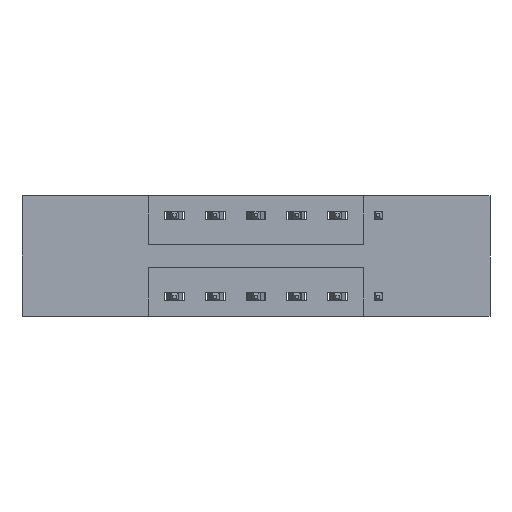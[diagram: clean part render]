
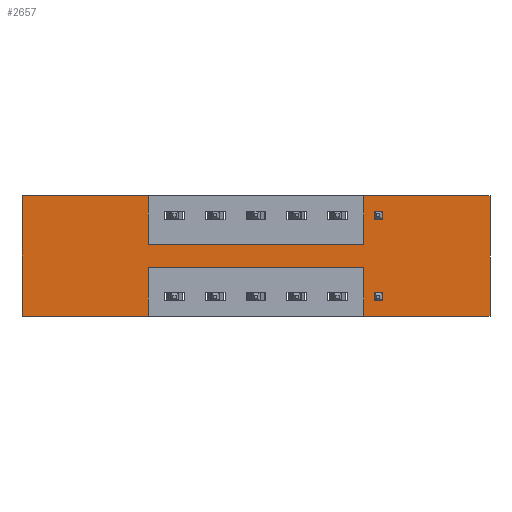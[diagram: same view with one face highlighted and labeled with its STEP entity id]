
A CAD part, front view. The second image highlights one B-rep face of the part: STEP entity #2657.
In plain terms, the highlighted planar face has unit normal (0, -1, 0).
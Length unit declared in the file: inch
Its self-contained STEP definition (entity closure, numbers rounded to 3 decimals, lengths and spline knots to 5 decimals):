
#103 = EDGE_CURVE ( 'NONE', #3690, #7489, #5145, .T. ) ;
#227 = LINE ( 'NONE', #2023, #5489 ) ;
#377 = CARTESIAN_POINT ( 'NONE',  ( 1.0475, 0., -0.37 ) ) ;
#405 = ORIENTED_EDGE ( 'NONE', *, *, #7038, .F. ) ;
#437 = VERTEX_POINT ( 'NONE', #2454 ) ;
#628 = LINE ( 'NONE', #7731, #2457 ) ;
#719 = CARTESIAN_POINT ( 'NONE',  ( 0., 0., -0.37 ) ) ;
#747 = CARTESIAN_POINT ( 'NONE',  ( 0.3875, 0., -0.22 ) ) ;
#749 = EDGE_CURVE ( 'NONE', #3052, #5755, #6843, .T. ) ;
#815 = VECTOR ( 'NONE', #6853, 39.37008 ) ;
#986 = CARTESIAN_POINT ( 'NONE',  ( 0.3875, 0., 0. ) ) ;
#1021 = ORIENTED_EDGE ( 'NONE', *, *, #3793, .F. ) ;
#1059 = LINE ( 'NONE', #377, #2829 ) ;
#1305 = ORIENTED_EDGE ( 'NONE', *, *, #3811, .F. ) ;
#1348 = VECTOR ( 'NONE', #4289, 39.37008 ) ;
#1505 = ORIENTED_EDGE ( 'NONE', *, *, #5177, .F. ) ;
#1814 = CARTESIAN_POINT ( 'NONE',  ( 1.0475, 0., 0. ) ) ;
#1896 = VERTEX_POINT ( 'NONE', #7807 ) ;
#1995 = FACE_OUTER_BOUND ( 'NONE', #5633, .T. ) ;
#2023 = CARTESIAN_POINT ( 'NONE',  ( 0., 0., -0.37 ) ) ;
#2025 = LINE ( 'NONE', #7241, #3007 ) ;
#2126 = EDGE_CURVE ( 'NONE', #5675, #1896, #7620, .T. ) ;
#2211 = EDGE_CURVE ( 'NONE', #4249, #5675, #4907, .T. ) ;
#2221 = DIRECTION ( 'NONE',  ( 1., 0., 0. ) ) ;
#2454 = CARTESIAN_POINT ( 'NONE',  ( 1.435, 0., 0. ) ) ;
#2457 = VECTOR ( 'NONE', #8298, 39.37008 ) ;
#2488 = DIRECTION ( 'NONE',  ( 0., 0., 1. ) ) ;
#2521 = LINE ( 'NONE', #3202, #1348 ) ;
#2657 = ADVANCED_FACE ( 'NONE', ( #1995 ), #7123, .T. ) ;
#2673 = VERTEX_POINT ( 'NONE', #7170 ) ;
#2764 = DIRECTION ( 'NONE',  ( -1., 0., 0. ) ) ;
#2829 = VECTOR ( 'NONE', #3634, 39.37008 ) ;
#2923 = EDGE_CURVE ( 'NONE', #3695, #2673, #227, .T. ) ;
#3007 = VECTOR ( 'NONE', #4045, 39.37008 ) ;
#3041 = VERTEX_POINT ( 'NONE', #747 ) ;
#3052 = VERTEX_POINT ( 'NONE', #8069 ) ;
#3202 = CARTESIAN_POINT ( 'NONE',  ( 0.3875, 0., -0.15 ) ) ;
#3571 = ORIENTED_EDGE ( 'NONE', *, *, #7753, .F. ) ;
#3614 = CARTESIAN_POINT ( 'NONE',  ( 0., 0., 0. ) ) ;
#3634 = DIRECTION ( 'NONE',  ( 0., 0., 1. ) ) ;
#3690 = VERTEX_POINT ( 'NONE', #986 ) ;
#3695 = VERTEX_POINT ( 'NONE', #7357 ) ;
#3751 = VECTOR ( 'NONE', #2221, 39.37008 ) ;
#3793 = EDGE_CURVE ( 'NONE', #6405, #3041, #7319, .T. ) ;
#3811 = EDGE_CURVE ( 'NONE', #1896, #3690, #5405, .T. ) ;
#4042 = DIRECTION ( 'NONE',  ( -1., 0., 0. ) ) ;
#4045 = DIRECTION ( 'NONE',  ( 0., 0., -1. ) ) ;
#4065 = VECTOR ( 'NONE', #2488, 39.37008 ) ;
#4086 = CARTESIAN_POINT ( 'NONE',  ( 0., 0., -0.37 ) ) ;
#4231 = VECTOR ( 'NONE', #8191, 39.37008 ) ;
#4249 = VERTEX_POINT ( 'NONE', #7999 ) ;
#4289 = DIRECTION ( 'NONE',  ( 1., 0., 0. ) ) ;
#4307 = CARTESIAN_POINT ( 'NONE',  ( 0.3875, 0., -0.15 ) ) ;
#4402 = CARTESIAN_POINT ( 'NONE',  ( 0., 0., -0.37 ) ) ;
#4501 = ORIENTED_EDGE ( 'NONE', *, *, #103, .F. ) ;
#4569 = VECTOR ( 'NONE', #5225, 39.37008 ) ;
#4907 = LINE ( 'NONE', #4402, #8269 ) ;
#4944 = DIRECTION ( 'NONE',  ( -1., 0., 0. ) ) ;
#5092 = CARTESIAN_POINT ( 'NONE',  ( 1.0475, 0., 0. ) ) ;
#5137 = DIRECTION ( 'NONE',  ( 0., 0., -1. ) ) ;
#5145 = LINE ( 'NONE', #8347, #4569 ) ;
#5177 = EDGE_CURVE ( 'NONE', #3041, #4249, #6374, .T. ) ;
#5225 = DIRECTION ( 'NONE',  ( 0., 0., -1. ) ) ;
#5405 = LINE ( 'NONE', #7987, #3751 ) ;
#5489 = VECTOR ( 'NONE', #4042, 39.37008 ) ;
#5633 = EDGE_LOOP ( 'NONE', ( #1505, #1021, #405, #6823, #7181, #3571, #6627, #8344, #4501, #1305, #5636, #5846 ) ) ;
#5636 = ORIENTED_EDGE ( 'NONE', *, *, #2126, .F. ) ;
#5675 = VERTEX_POINT ( 'NONE', #4086 ) ;
#5755 = VERTEX_POINT ( 'NONE', #5092 ) ;
#5846 = ORIENTED_EDGE ( 'NONE', *, *, #2211, .F. ) ;
#5950 = DIRECTION ( 'NONE',  ( 0., -1., 0. ) ) ;
#6032 = AXIS2_PLACEMENT_3D ( 'NONE', #719, #5950, #5137 ) ;
#6048 = CARTESIAN_POINT ( 'NONE',  ( 0.3875, 0., -0.22 ) ) ;
#6374 = LINE ( 'NONE', #8338, #815 ) ;
#6382 = EDGE_CURVE ( 'NONE', #7489, #3052, #2521, .T. ) ;
#6405 = VERTEX_POINT ( 'NONE', #7628 ) ;
#6625 = EDGE_CURVE ( 'NONE', #437, #3695, #2025, .T. ) ;
#6627 = ORIENTED_EDGE ( 'NONE', *, *, #749, .F. ) ;
#6823 = ORIENTED_EDGE ( 'NONE', *, *, #2923, .F. ) ;
#6843 = LINE ( 'NONE', #1814, #4065 ) ;
#6853 = DIRECTION ( 'NONE',  ( 0., 0., -1. ) ) ;
#7038 = EDGE_CURVE ( 'NONE', #2673, #6405, #1059, .T. ) ;
#7123 = PLANE ( 'NONE',  #6032 ) ;
#7170 = CARTESIAN_POINT ( 'NONE',  ( 1.0475, 0., -0.37 ) ) ;
#7181 = ORIENTED_EDGE ( 'NONE', *, *, #6625, .F. ) ;
#7241 = CARTESIAN_POINT ( 'NONE',  ( 1.435, 0., 0. ) ) ;
#7319 = LINE ( 'NONE', #6048, #8060 ) ;
#7357 = CARTESIAN_POINT ( 'NONE',  ( 1.435, 0., -0.37 ) ) ;
#7489 = VERTEX_POINT ( 'NONE', #4307 ) ;
#7620 = LINE ( 'NONE', #3614, #4231 ) ;
#7628 = CARTESIAN_POINT ( 'NONE',  ( 1.0475, 0., -0.22 ) ) ;
#7731 = CARTESIAN_POINT ( 'NONE',  ( 0., 0., 0. ) ) ;
#7753 = EDGE_CURVE ( 'NONE', #5755, #437, #628, .T. ) ;
#7807 = CARTESIAN_POINT ( 'NONE',  ( 0., 0., 0. ) ) ;
#7987 = CARTESIAN_POINT ( 'NONE',  ( 0., 0., 0. ) ) ;
#7999 = CARTESIAN_POINT ( 'NONE',  ( 0.3875, 0., -0.37 ) ) ;
#8060 = VECTOR ( 'NONE', #2764, 39.37008 ) ;
#8069 = CARTESIAN_POINT ( 'NONE',  ( 1.0475, 0., -0.15 ) ) ;
#8191 = DIRECTION ( 'NONE',  ( 0., 0., 1. ) ) ;
#8269 = VECTOR ( 'NONE', #4944, 39.37008 ) ;
#8298 = DIRECTION ( 'NONE',  ( 1., 0., 0. ) ) ;
#8338 = CARTESIAN_POINT ( 'NONE',  ( 0.3875, 0., -0.37 ) ) ;
#8344 = ORIENTED_EDGE ( 'NONE', *, *, #6382, .F. ) ;
#8347 = CARTESIAN_POINT ( 'NONE',  ( 0.3875, 0., 0. ) ) ;
